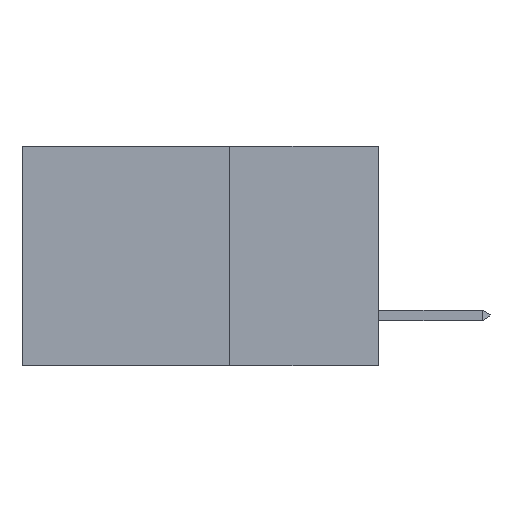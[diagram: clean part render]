
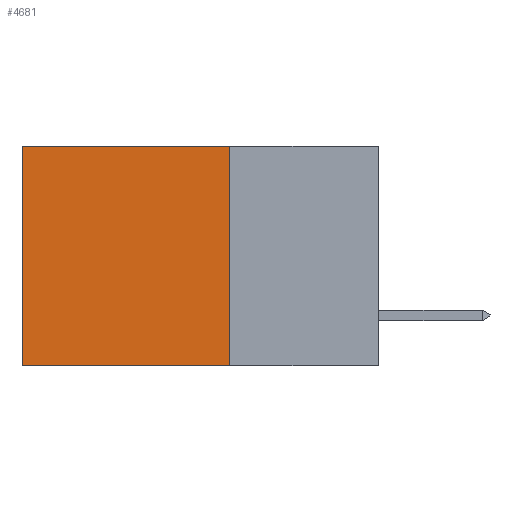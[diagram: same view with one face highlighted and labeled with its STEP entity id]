
A CAD part, left-side view. The second image highlights one B-rep face of the part: STEP entity #4681.
In plain terms, the highlighted planar face has unit normal (-1, 0, 0).
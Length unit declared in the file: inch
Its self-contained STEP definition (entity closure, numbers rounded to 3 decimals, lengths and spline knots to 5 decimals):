
#450 = ORIENTED_EDGE ( 'NONE', *, *, #8167, .F. ) ;
#2203 = PLANE ( 'NONE',  #5334 ) ;
#3165 = VERTEX_POINT ( 'NONE', #5587 ) ;
#3823 = LINE ( 'NONE', #6263, #9616 ) ;
#4136 = CARTESIAN_POINT ( 'NONE',  ( 0.2615, 0.25, -0.37 ) ) ;
#4537 = LINE ( 'NONE', #8178, #4692 ) ;
#4681 = ADVANCED_FACE ( 'NONE', ( #7529 ), #2203, .F. ) ;
#4692 = VECTOR ( 'NONE', #8034, 39.37008 ) ;
#4863 = VERTEX_POINT ( 'NONE', #5014 ) ;
#4920 = EDGE_CURVE ( 'NONE', #4923, #3165, #3823, .T. ) ;
#4923 = VERTEX_POINT ( 'NONE', #5306 ) ;
#5014 = CARTESIAN_POINT ( 'NONE',  ( 0.2615, 0.25, 0. ) ) ;
#5198 = DIRECTION ( 'NONE',  ( 0., 1., 0. ) ) ;
#5306 = CARTESIAN_POINT ( 'NONE',  ( 0.2615, 0.6, 0. ) ) ;
#5334 = AXIS2_PLACEMENT_3D ( 'NONE', #14205, #12984, #9874 ) ;
#5463 = CARTESIAN_POINT ( 'NONE',  ( 0.2615, 0.25, -0.37 ) ) ;
#5587 = CARTESIAN_POINT ( 'NONE',  ( 0.2615, 0.6, -0.37 ) ) ;
#6091 = VECTOR ( 'NONE', #12873, 39.37008 ) ;
#6184 = EDGE_CURVE ( 'NONE', #4863, #4923, #6650, .T. ) ;
#6263 = CARTESIAN_POINT ( 'NONE',  ( 0.2615, 0.6, -0.37 ) ) ;
#6308 = EDGE_LOOP ( 'NONE', ( #11507, #450, #8280, #8577 ) ) ;
#6650 = LINE ( 'NONE', #10664, #7837 ) ;
#7529 = FACE_OUTER_BOUND ( 'NONE', #6308, .T. ) ;
#7837 = VECTOR ( 'NONE', #5198, 39.37008 ) ;
#8034 = DIRECTION ( 'NONE',  ( 0., 0., -1. ) ) ;
#8167 = EDGE_CURVE ( 'NONE', #13373, #3165, #12596, .T. ) ;
#8178 = CARTESIAN_POINT ( 'NONE',  ( 0.2615, 0.25, -0.37 ) ) ;
#8280 = ORIENTED_EDGE ( 'NONE', *, *, #12159, .F. ) ;
#8577 = ORIENTED_EDGE ( 'NONE', *, *, #6184, .T. ) ;
#9616 = VECTOR ( 'NONE', #11777, 39.37008 ) ;
#9874 = DIRECTION ( 'NONE',  ( 0., 0., -1. ) ) ;
#10664 = CARTESIAN_POINT ( 'NONE',  ( 0.2615, 0.25, 0. ) ) ;
#11507 = ORIENTED_EDGE ( 'NONE', *, *, #4920, .T. ) ;
#11777 = DIRECTION ( 'NONE',  ( 0., 0., -1. ) ) ;
#12159 = EDGE_CURVE ( 'NONE', #4863, #13373, #4537, .T. ) ;
#12596 = LINE ( 'NONE', #4136, #6091 ) ;
#12873 = DIRECTION ( 'NONE',  ( 0., 1., 0. ) ) ;
#12984 = DIRECTION ( 'NONE',  ( 1., 0., 0. ) ) ;
#13373 = VERTEX_POINT ( 'NONE', #5463 ) ;
#14205 = CARTESIAN_POINT ( 'NONE',  ( 0.2615, 0.25, -0.37 ) ) ;
